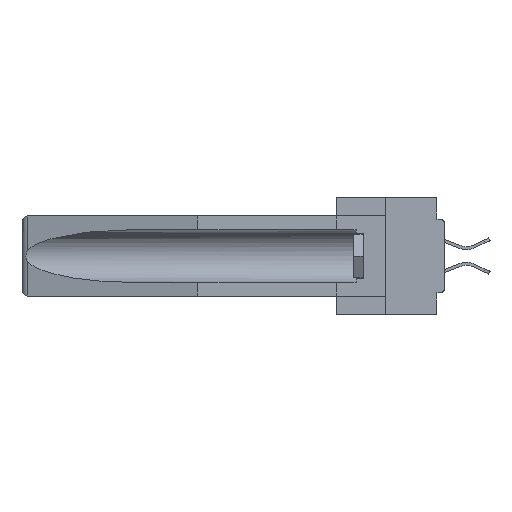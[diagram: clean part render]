
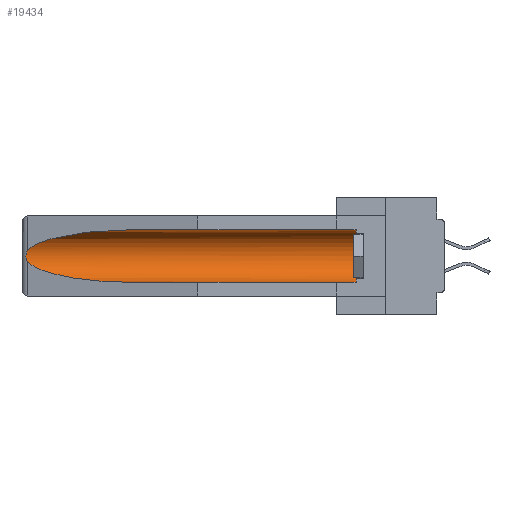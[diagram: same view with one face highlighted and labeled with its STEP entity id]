
A CAD part, left-side view. The second image highlights one B-rep face of the part: STEP entity #19434.
In plain terms, the highlighted cylindrical face has radius 2.857 mm (diameter 5.715 mm), a partial arc.
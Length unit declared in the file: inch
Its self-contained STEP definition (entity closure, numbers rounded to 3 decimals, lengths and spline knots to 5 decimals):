
#967 = EDGE_CURVE ( 'NONE', #9436, #25045, #42933, .T. ) ;
#1012 = CARTESIAN_POINT ( 'NONE',  ( 0.155, 1.07973, -0.284 ) ) ;
#2176 = CARTESIAN_POINT ( 'NONE',  ( 0.26537, 1.52718, -0.19328 ) ) ;
#4005 = CARTESIAN_POINT ( 'NONE',  ( 0.26537, 1.52718, -0.14972 ) ) ;
#4309 = CYLINDRICAL_SURFACE ( 'NONE', #6392, 0.1125 ) ;
#4453 = ORIENTED_EDGE ( 'NONE', *, *, #8898, .T. ) ;
#4864 = CARTESIAN_POINT ( 'NONE',  ( 0.155, 0.126, -0.059 ) ) ;
#5013 = CARTESIAN_POINT ( 'NONE',  ( 0.26654, 1.53092, -0.15636 ) ) ;
#5871 = FACE_OUTER_BOUND ( 'NONE', #20663, .T. ) ;
#6170 = CARTESIAN_POINT ( 'NONE',  ( 0.155, 1.07973, -0.059 ) ) ;
#6273 = DIRECTION ( 'NONE',  ( 0., 1., 0. ) ) ;
#6392 = AXIS2_PLACEMENT_3D ( 'NONE', #13939, #41566, #14392 ) ;
#8898 = EDGE_CURVE ( 'NONE', #25045, #15537, #17177, .T. ) ;
#8903 = CARTESIAN_POINT ( 'NONE',  ( 0.26537, 1.52718, -0.14972 ) ) ;
#9436 = VERTEX_POINT ( 'NONE', #4864 ) ;
#10096 = ORIENTED_EDGE ( 'NONE', *, *, #16649, .T. ) ;
#10591 = B_SPLINE_CURVE_WITH_KNOTS ( 'NONE', 3,
 ( #8903, #18777, #5013, #36423, #12369, #22035, #28872, #25762, #36267, #2176 ),
 .UNSPECIFIED., .F., .F.,
 ( 4, 2, 2, 2, 4 ),
 ( 0., 0.00029, 0.00058, 0.00087, 0.00117 ),
 .UNSPECIFIED. ) ;
#11194 = CARTESIAN_POINT ( 'NONE',  ( 0.26537, 1.52718, -0.14972 ) ) ;
#12369 = CARTESIAN_POINT ( 'NONE',  ( 0.2675, 1.53308, -0.16763 ) ) ;
#13001 = VERTEX_POINT ( 'NONE', #20491 ) ;
#13939 = CARTESIAN_POINT ( 'NONE',  ( 0.155, -0.30754, -0.1715 ) ) ;
#14073 = CARTESIAN_POINT ( 'NONE',  ( 0.25451, 1.48313, -0.09465 ) ) ;
#14392 = DIRECTION ( 'NONE',  ( 0., 0., 1. ) ) ;
#14537 = CARTESIAN_POINT ( 'NONE',  ( 0.155, 1.07973, -0.059 ) ) ;
#14631 = CARTESIAN_POINT ( 'NONE',  ( 0.155, 0.126, -0.1715 ) ) ;
#15537 = VERTEX_POINT ( 'NONE', #11194 ) ;
#16047 = DIRECTION ( 'NONE',  ( 0., 1., 0. ) ) ;
#16649 = EDGE_CURVE ( 'NONE', #13001, #41364, #41596, .T. ) ;
#16723 = CARTESIAN_POINT ( 'NONE',  ( 0.155, -0.30754, -0.284 ) ) ;
#17177 =( BOUNDED_CURVE ( )  B_SPLINE_CURVE ( 3, ( #14537, #24169, #14073, #4005 ),
 .UNSPECIFIED., .F., .F. ) 
 B_SPLINE_CURVE_WITH_KNOTS ( ( 4, 4 ),
 ( 4.71239, 6.08839 ),
 .UNSPECIFIED. ) 
 CURVE ( )  GEOMETRIC_REPRESENTATION_ITEM ( )  RATIONAL_B_SPLINE_CURVE ( ( 1., 0.848, 0.848, 1. ) ) 
 REPRESENTATION_ITEM ( '' )  );
#18777 = CARTESIAN_POINT ( 'NONE',  ( 0.26597, 1.52961, -0.15275 ) ) ;
#19434 = ADVANCED_FACE ( 'NONE', ( #5871 ), #4309, .F. ) ;
#20491 = CARTESIAN_POINT ( 'NONE',  ( 0.26537, 1.52718, -0.19328 ) ) ;
#20663 = EDGE_LOOP ( 'NONE', ( #4453, #41304, #10096, #35051, #41623, #30396 ) ) ;
#22035 = CARTESIAN_POINT ( 'NONE',  ( 0.2675, 1.53308, -0.17534 ) ) ;
#23220 = EDGE_CURVE ( 'NONE', #26859, #9436, #29985, .T. ) ;
#23404 = EDGE_CURVE ( 'NONE', #15537, #13001, #10591, .T. ) ;
#24169 = CARTESIAN_POINT ( 'NONE',  ( 0.21114, 1.30732, -0.059 ) ) ;
#25045 = VERTEX_POINT ( 'NONE', #6170 ) ;
#25762 = CARTESIAN_POINT ( 'NONE',  ( 0.26655, 1.53094, -0.18657 ) ) ;
#26859 = VERTEX_POINT ( 'NONE', #43514 ) ;
#28137 = CARTESIAN_POINT ( 'NONE',  ( 0.25451, 1.48313, -0.24835 ) ) ;
#28872 = CARTESIAN_POINT ( 'NONE',  ( 0.2673, 1.53269, -0.17917 ) ) ;
#28901 = VECTOR ( 'NONE', #6273, 39.37008 ) ;
#29960 = EDGE_CURVE ( 'NONE', #26859, #41364, #31047, .T. ) ;
#29985 = CIRCLE ( 'NONE', #42907, 0.1125 ) ;
#30396 = ORIENTED_EDGE ( 'NONE', *, *, #967, .T. ) ;
#31047 = LINE ( 'NONE', #16723, #28901 ) ;
#34021 = CARTESIAN_POINT ( 'NONE',  ( 0.155, 1.07973, -0.284 ) ) ;
#34942 = CARTESIAN_POINT ( 'NONE',  ( 0.26537, 1.52718, -0.19328 ) ) ;
#35051 = ORIENTED_EDGE ( 'NONE', *, *, #29960, .F. ) ;
#36267 = CARTESIAN_POINT ( 'NONE',  ( 0.26597, 1.5296, -0.19026 ) ) ;
#36423 = CARTESIAN_POINT ( 'NONE',  ( 0.2673, 1.5327, -0.16383 ) ) ;
#40386 = CARTESIAN_POINT ( 'NONE',  ( 0.155, -0.30754, -0.059 ) ) ;
#41304 = ORIENTED_EDGE ( 'NONE', *, *, #23404, .T. ) ;
#41364 = VERTEX_POINT ( 'NONE', #34021 ) ;
#41566 = DIRECTION ( 'NONE',  ( 0., 1., 0. ) ) ;
#41596 =( BOUNDED_CURVE ( )  B_SPLINE_CURVE ( 3, ( #34942, #28137, #42286, #1012 ),
 .UNSPECIFIED., .F., .F. ) 
 B_SPLINE_CURVE_WITH_KNOTS ( ( 4, 4 ),
 ( 0.1948, 1.5708 ),
 .UNSPECIFIED. ) 
 CURVE ( )  GEOMETRIC_REPRESENTATION_ITEM ( )  RATIONAL_B_SPLINE_CURVE ( ( 1., 0.848, 0.848, 1. ) ) 
 REPRESENTATION_ITEM ( '' )  );
#41623 = ORIENTED_EDGE ( 'NONE', *, *, #23220, .T. ) ;
#41957 = DIRECTION ( 'NONE',  ( 0., 0., 1. ) ) ;
#42264 = DIRECTION ( 'NONE',  ( 0., -1., 0. ) ) ;
#42286 = CARTESIAN_POINT ( 'NONE',  ( 0.21114, 1.30732, -0.284 ) ) ;
#42907 = AXIS2_PLACEMENT_3D ( 'NONE', #14631, #42264, #41957 ) ;
#42933 = LINE ( 'NONE', #40386, #43446 ) ;
#43446 = VECTOR ( 'NONE', #16047, 39.37008 ) ;
#43514 = CARTESIAN_POINT ( 'NONE',  ( 0.155, 0.126, -0.284 ) ) ;
